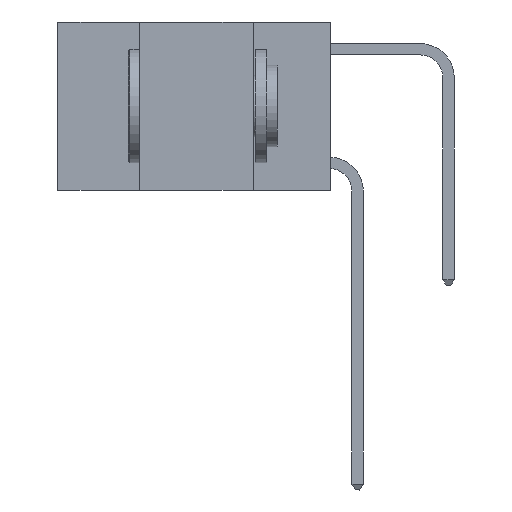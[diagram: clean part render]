
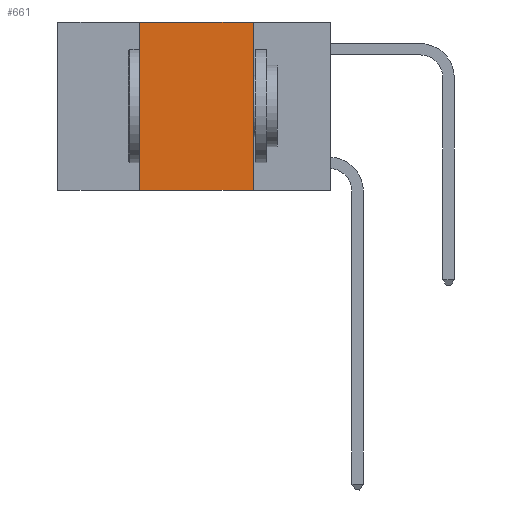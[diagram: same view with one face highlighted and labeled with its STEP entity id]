
A CAD part, left-side view. The second image highlights one B-rep face of the part: STEP entity #661.
In plain terms, the highlighted planar face has unit normal (-1, 0, 0).
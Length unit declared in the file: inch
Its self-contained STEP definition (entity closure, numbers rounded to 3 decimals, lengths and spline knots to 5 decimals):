
#130 = VERTEX_POINT ( 'NONE', #4923 ) ;
#248 = DIRECTION ( 'NONE',  ( 0., -1., 0. ) ) ;
#403 = CARTESIAN_POINT ( 'NONE',  ( 0., 0.42, -0.37 ) ) ;
#425 = LINE ( 'NONE', #8995, #2525 ) ;
#661 = ADVANCED_FACE ( 'NONE', ( #12602 ), #12844, .F. ) ;
#971 = VERTEX_POINT ( 'NONE', #403 ) ;
#1394 = DIRECTION ( 'NONE',  ( 0., 0., 1. ) ) ;
#1475 = DIRECTION ( 'NONE',  ( 0., -1., 0. ) ) ;
#1703 = CARTESIAN_POINT ( 'NONE',  ( 0., 0.6, 0. ) ) ;
#1812 = EDGE_CURVE ( 'NONE', #6109, #130, #2806, .T. ) ;
#2090 = DIRECTION ( 'NONE',  ( 0., 0., -1. ) ) ;
#2525 = VECTOR ( 'NONE', #11838, 39.37008 ) ;
#2806 = LINE ( 'NONE', #1703, #6452 ) ;
#3505 = EDGE_LOOP ( 'NONE', ( #8387, #8623, #8861, #8962 ) ) ;
#3926 = LINE ( 'NONE', #4324, #9018 ) ;
#4324 = CARTESIAN_POINT ( 'NONE',  ( 0., 0.6, -0.37 ) ) ;
#4352 = CARTESIAN_POINT ( 'NONE',  ( 0., 0.42, 0. ) ) ;
#4923 = CARTESIAN_POINT ( 'NONE',  ( 0., 0.17, 0. ) ) ;
#5517 = EDGE_CURVE ( 'NONE', #971, #6109, #9822, .T. ) ;
#5636 = CARTESIAN_POINT ( 'NONE',  ( 0., 0.6, 0. ) ) ;
#5981 = DIRECTION ( 'NONE',  ( 1., 0., 0. ) ) ;
#6033 = CARTESIAN_POINT ( 'NONE',  ( 0., 0.17, -0.37 ) ) ;
#6109 = VERTEX_POINT ( 'NONE', #4352 ) ;
#6452 = VECTOR ( 'NONE', #1475, 39.37008 ) ;
#6584 = VERTEX_POINT ( 'NONE', #6033 ) ;
#7182 = VECTOR ( 'NONE', #1394, 39.37008 ) ;
#8387 = ORIENTED_EDGE ( 'NONE', *, *, #9377, .F. ) ;
#8558 = AXIS2_PLACEMENT_3D ( 'NONE', #5636, #5981, #2090 ) ;
#8623 = ORIENTED_EDGE ( 'NONE', *, *, #1812, .F. ) ;
#8861 = ORIENTED_EDGE ( 'NONE', *, *, #5517, .F. ) ;
#8962 = ORIENTED_EDGE ( 'NONE', *, *, #11624, .T. ) ;
#8995 = CARTESIAN_POINT ( 'NONE',  ( 0., 0.17, 0. ) ) ;
#9018 = VECTOR ( 'NONE', #248, 39.37008 ) ;
#9377 = EDGE_CURVE ( 'NONE', #130, #6584, #425, .T. ) ;
#9822 = LINE ( 'NONE', #11389, #7182 ) ;
#11389 = CARTESIAN_POINT ( 'NONE',  ( 0., 0.42, 0. ) ) ;
#11624 = EDGE_CURVE ( 'NONE', #971, #6584, #3926, .T. ) ;
#11838 = DIRECTION ( 'NONE',  ( 0., 0., -1. ) ) ;
#12602 = FACE_OUTER_BOUND ( 'NONE', #3505, .T. ) ;
#12844 = PLANE ( 'NONE',  #8558 ) ;
